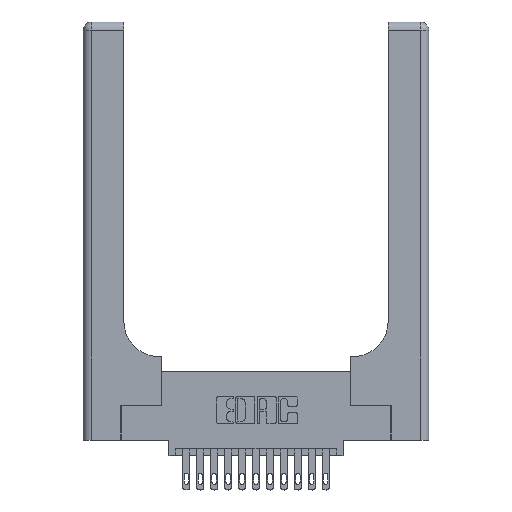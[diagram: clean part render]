
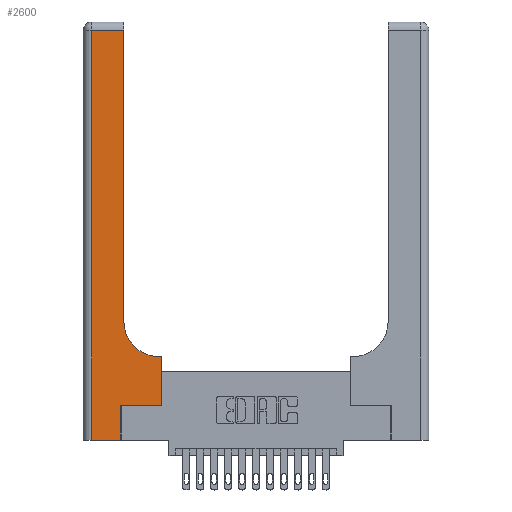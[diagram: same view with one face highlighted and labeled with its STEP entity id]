
A CAD part, top view. The second image highlights one B-rep face of the part: STEP entity #2600.
In plain terms, the highlighted planar face has unit normal (0, 0, 1).
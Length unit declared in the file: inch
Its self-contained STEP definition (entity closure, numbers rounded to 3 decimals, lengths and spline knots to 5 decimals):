
#77 = PLANE ( 'NONE',  #17735 ) ;
#84 = DIRECTION ( 'NONE',  ( 1., 0., 0. ) ) ;
#96 = VECTOR ( 'NONE', #12350, 39.37008 ) ;
#283 = LINE ( 'NONE', #15030, #8144 ) ;
#471 = LINE ( 'NONE', #6351, #10254 ) ;
#809 = EDGE_CURVE ( 'NONE', #18029, #13351, #283, .T. ) ;
#987 = EDGE_CURVE ( 'NONE', #15005, #7667, #15698, .T. ) ;
#1562 = DIRECTION ( 'NONE',  ( 0., 0., -1. ) ) ;
#1652 = VECTOR ( 'NONE', #4317, 39.37008 ) ;
#2032 = ORIENTED_EDGE ( 'NONE', *, *, #809, .T. ) ;
#2305 = VERTEX_POINT ( 'NONE', #5498 ) ;
#2315 = DIRECTION ( 'NONE',  ( 1., 0., 0. ) ) ;
#2447 = VECTOR ( 'NONE', #17657, 39.37008 ) ;
#2479 = VERTEX_POINT ( 'NONE', #9606 ) ;
#2531 = LINE ( 'NONE', #9729, #1652 ) ;
#2600 = ADVANCED_FACE ( 'NONE', ( #17586 ), #77, .F. ) ;
#2891 = CARTESIAN_POINT ( 'NONE',  ( 0., 3., 0.37 ) ) ;
#3085 = EDGE_CURVE ( 'NONE', #2305, #16375, #2531, .T. ) ;
#3119 = LINE ( 'NONE', #4850, #17500 ) ;
#3157 = CARTESIAN_POINT ( 'NONE',  ( 0.5585, 0.25, 0.37 ) ) ;
#3302 = VERTEX_POINT ( 'NONE', #5579 ) ;
#3369 = EDGE_CURVE ( 'NONE', #16375, #2479, #3394, .T. ) ;
#3394 = LINE ( 'NONE', #11144, #13588 ) ;
#3587 = DIRECTION ( 'NONE',  ( 0., 1., 0. ) ) ;
#4143 = EDGE_CURVE ( 'NONE', #7667, #9309, #17519, .T. ) ;
#4317 = DIRECTION ( 'NONE',  ( 0., -1., 0. ) ) ;
#4693 = ORIENTED_EDGE ( 'NONE', *, *, #4143, .T. ) ;
#4850 = CARTESIAN_POINT ( 'NONE',  ( 0.2915, 0.6, 0.37 ) ) ;
#4963 = DIRECTION ( 'NONE',  ( -1., 0., 0. ) ) ;
#5140 = EDGE_CURVE ( 'NONE', #3302, #15005, #3119, .T. ) ;
#5150 = LINE ( 'NONE', #17879, #96 ) ;
#5493 = ORIENTED_EDGE ( 'NONE', *, *, #5140, .T. ) ;
#5498 = CARTESIAN_POINT ( 'NONE',  ( 0.06, 2.94, 0.37 ) ) ;
#5579 = CARTESIAN_POINT ( 'NONE',  ( 0.5585, 0.6, 0.37 ) ) ;
#6224 = VECTOR ( 'NONE', #8523, 39.37008 ) ;
#6351 = CARTESIAN_POINT ( 'NONE',  ( 0.269, 0., 0.37 ) ) ;
#6871 = DIRECTION ( 'NONE',  ( -1., 0., 0. ) ) ;
#6959 = EDGE_CURVE ( 'NONE', #2479, #18029, #471, .T. ) ;
#7667 = VERTEX_POINT ( 'NONE', #10340 ) ;
#7813 = CARTESIAN_POINT ( 'NONE',  ( 0.269, 0.25, 0.37 ) ) ;
#8144 = VECTOR ( 'NONE', #2315, 39.37008 ) ;
#8523 = DIRECTION ( 'NONE',  ( 0., 1., 0. ) ) ;
#8558 = ORIENTED_EDGE ( 'NONE', *, *, #3369, .T. ) ;
#9191 = LINE ( 'NONE', #14661, #2447 ) ;
#9309 = VERTEX_POINT ( 'NONE', #12875 ) ;
#9428 = ORIENTED_EDGE ( 'NONE', *, *, #18014, .T. ) ;
#9509 = CARTESIAN_POINT ( 'NONE',  ( 0.06, 0., 0.37 ) ) ;
#9606 = CARTESIAN_POINT ( 'NONE',  ( 0.269, 0., 0.37 ) ) ;
#9729 = CARTESIAN_POINT ( 'NONE',  ( 0.06, 3., 0.37 ) ) ;
#10254 = VECTOR ( 'NONE', #3587, 39.37008 ) ;
#10340 = CARTESIAN_POINT ( 'NONE',  ( 0.2915, 0.85, 0.37 ) ) ;
#10445 = AXIS2_PLACEMENT_3D ( 'NONE', #17848, #11232, #12620 ) ;
#11144 = CARTESIAN_POINT ( 'NONE',  ( 0., 0., 0.37 ) ) ;
#11231 = CARTESIAN_POINT ( 'NONE',  ( 0.5415, 0.6, 0.37 ) ) ;
#11232 = DIRECTION ( 'NONE',  ( 0., 0., -1. ) ) ;
#12350 = DIRECTION ( 'NONE',  ( 0., 1., 0. ) ) ;
#12620 = DIRECTION ( 'NONE',  ( 1., 0., 0. ) ) ;
#12875 = CARTESIAN_POINT ( 'NONE',  ( 0.2915, 2.94, 0.37 ) ) ;
#12886 = EDGE_LOOP ( 'NONE', ( #4693, #9428, #15791, #8558, #13466, #2032, #16807, #5493, #15520 ) ) ;
#13351 = VERTEX_POINT ( 'NONE', #3157 ) ;
#13466 = ORIENTED_EDGE ( 'NONE', *, *, #6959, .T. ) ;
#13588 = VECTOR ( 'NONE', #84, 39.37008 ) ;
#14081 = CARTESIAN_POINT ( 'NONE',  ( 0.2915, 3., 0.37 ) ) ;
#14661 = CARTESIAN_POINT ( 'NONE',  ( 0., 2.94, 0.37 ) ) ;
#15005 = VERTEX_POINT ( 'NONE', #11231 ) ;
#15030 = CARTESIAN_POINT ( 'NONE',  ( 0.269, 0.25, 0.37 ) ) ;
#15520 = ORIENTED_EDGE ( 'NONE', *, *, #987, .T. ) ;
#15587 = EDGE_CURVE ( 'NONE', #13351, #3302, #5150, .T. ) ;
#15698 = CIRCLE ( 'NONE', #10445, 0.25 ) ;
#15791 = ORIENTED_EDGE ( 'NONE', *, *, #3085, .T. ) ;
#16375 = VERTEX_POINT ( 'NONE', #9509 ) ;
#16807 = ORIENTED_EDGE ( 'NONE', *, *, #15587, .T. ) ;
#17500 = VECTOR ( 'NONE', #4963, 39.37008 ) ;
#17519 = LINE ( 'NONE', #14081, #6224 ) ;
#17586 = FACE_OUTER_BOUND ( 'NONE', #12886, .T. ) ;
#17657 = DIRECTION ( 'NONE',  ( -1., 0., 0. ) ) ;
#17735 = AXIS2_PLACEMENT_3D ( 'NONE', #2891, #1562, #6871 ) ;
#17848 = CARTESIAN_POINT ( 'NONE',  ( 0.5415, 0.85, 0.37 ) ) ;
#17879 = CARTESIAN_POINT ( 'NONE',  ( 0.5585, 0.25, 0.37 ) ) ;
#18014 = EDGE_CURVE ( 'NONE', #9309, #2305, #9191, .T. ) ;
#18029 = VERTEX_POINT ( 'NONE', #7813 ) ;
